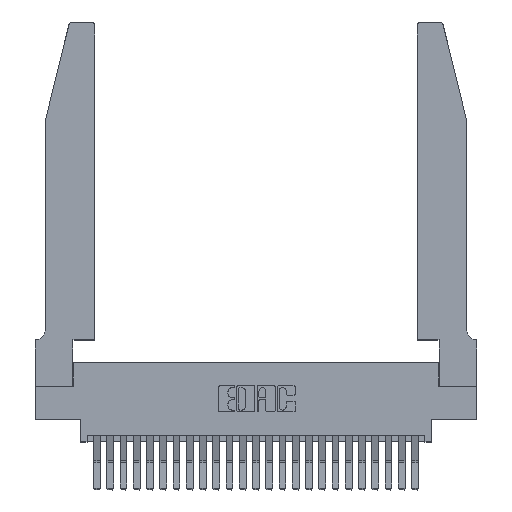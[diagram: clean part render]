
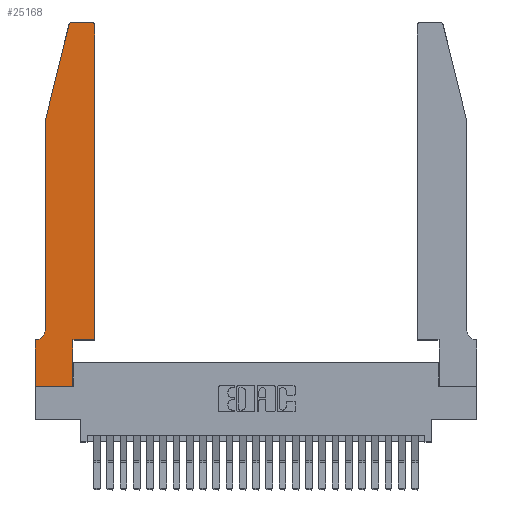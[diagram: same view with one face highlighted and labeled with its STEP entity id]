
A CAD part, top view. The second image highlights one B-rep face of the part: STEP entity #25168.
In plain terms, the highlighted planar face has unit normal (0, 0, 1).
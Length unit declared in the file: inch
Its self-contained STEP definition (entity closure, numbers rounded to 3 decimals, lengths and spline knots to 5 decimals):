
#129 = ORIENTED_EDGE ( 'NONE', *, *, #20044, .T. ) ;
#141 = EDGE_CURVE ( 'NONE', #10245, #15289, #26873, .T. ) ;
#206 = VERTEX_POINT ( 'NONE', #9974 ) ;
#524 = VERTEX_POINT ( 'NONE', #25598 ) ;
#725 = DIRECTION ( 'NONE',  ( 0., -1., 0. ) ) ;
#906 = LINE ( 'NONE', #17146, #22350 ) ;
#1101 = DIRECTION ( 'NONE',  ( 1., 0., 0. ) ) ;
#1285 = CARTESIAN_POINT ( 'NONE',  ( 0., 0., 0.37 ) ) ;
#1802 = DIRECTION ( 'NONE',  ( 1., 0., 0. ) ) ;
#1846 = DIRECTION ( 'NONE',  ( 1., 0., 0. ) ) ;
#2119 = DIRECTION ( 'NONE',  ( 1., 0., 0. ) ) ;
#2257 = VERTEX_POINT ( 'NONE', #11259 ) ;
#2461 = VERTEX_POINT ( 'NONE', #10175 ) ;
#2646 = CARTESIAN_POINT ( 'NONE',  ( 0.2865, 0.35, 0.37 ) ) ;
#2958 = DIRECTION ( 'NONE',  ( 0., -1., 0. ) ) ;
#3102 = LINE ( 'NONE', #10733, #10569 ) ;
#3247 = DIRECTION ( 'NONE',  ( 0., 0., -1. ) ) ;
#3301 = VECTOR ( 'NONE', #19074, 39.37008 ) ;
#3328 = DIRECTION ( 'NONE',  ( -1., 0., 0. ) ) ;
#3573 = ORIENTED_EDGE ( 'NONE', *, *, #22292, .T. ) ;
#4058 = CARTESIAN_POINT ( 'NONE',  ( 0.2865, 0., 0.37 ) ) ;
#4176 = CARTESIAN_POINT ( 'NONE',  ( 0.284, 2.72, 0.37 ) ) ;
#4724 = DIRECTION ( 'NONE',  ( -1., 0., 0. ) ) ;
#5297 = EDGE_CURVE ( 'NONE', #2461, #15305, #26559, .T. ) ;
#6252 = DIRECTION ( 'NONE',  ( 0., 0., 1. ) ) ;
#6571 = LINE ( 'NONE', #19351, #14093 ) ;
#6821 = CARTESIAN_POINT ( 'NONE',  ( 0.0755, 2., 0.37 ) ) ;
#8067 = AXIS2_PLACEMENT_3D ( 'NONE', #9018, #15135, #12956 ) ;
#8421 = ORIENTED_EDGE ( 'NONE', *, *, #18943, .T. ) ;
#8515 = CIRCLE ( 'NONE', #12895, 0.03 ) ;
#8526 = ORIENTED_EDGE ( 'NONE', *, *, #15415, .T. ) ;
#9018 = CARTESIAN_POINT ( 'NONE',  ( 0., 0.35, 0.37 ) ) ;
#9131 = CARTESIAN_POINT ( 'NONE',  ( 0.4505, 0.35, 0.37 ) ) ;
#9262 = DIRECTION ( 'NONE',  ( -0.239, -0.971, 0. ) ) ;
#9376 = CARTESIAN_POINT ( 'NONE',  ( 0.0755, 2., 0.37 ) ) ;
#9525 = CARTESIAN_POINT ( 'NONE',  ( 0.4205, 2.72, 0.37 ) ) ;
#9974 = CARTESIAN_POINT ( 'NONE',  ( 0.4505, 2.72, 0.37 ) ) ;
#10175 = CARTESIAN_POINT ( 'NONE',  ( 0.25487, 2.72718, 0.37 ) ) ;
#10245 = VERTEX_POINT ( 'NONE', #1285 ) ;
#10316 = VERTEX_POINT ( 'NONE', #25135 ) ;
#10436 = ORIENTED_EDGE ( 'NONE', *, *, #25226, .T. ) ;
#10569 = VECTOR ( 'NONE', #17134, 39.37008 ) ;
#10733 = CARTESIAN_POINT ( 'NONE',  ( 0.2605, 2.75, 0.37 ) ) ;
#10948 = CARTESIAN_POINT ( 'NONE',  ( 0.0055, 0.35, 0.37 ) ) ;
#11096 = CARTESIAN_POINT ( 'NONE',  ( 0.4205, 2.75, 0.37 ) ) ;
#11259 = CARTESIAN_POINT ( 'NONE',  ( 0.2865, 0.35, 0.37 ) ) ;
#11508 = CARTESIAN_POINT ( 'NONE',  ( 0.0055, 0.42, 0.37 ) ) ;
#11611 = VECTOR ( 'NONE', #1802, 39.37008 ) ;
#12684 = CARTESIAN_POINT ( 'NONE',  ( 0.284, 2.75, 0.37 ) ) ;
#12704 = EDGE_CURVE ( 'NONE', #206, #19803, #8515, .T. ) ;
#12749 = FACE_OUTER_BOUND ( 'NONE', #19467, .T. ) ;
#12799 = LINE ( 'NONE', #18111, #26760 ) ;
#12869 = ORIENTED_EDGE ( 'NONE', *, *, #14591, .T. ) ;
#12895 = AXIS2_PLACEMENT_3D ( 'NONE', #9525, #13556, #1101 ) ;
#12956 = DIRECTION ( 'NONE',  ( 1., 0., 0. ) ) ;
#13161 = CARTESIAN_POINT ( 'NONE',  ( 0., 0., 0.37 ) ) ;
#13297 = EDGE_CURVE ( 'NONE', #15289, #2257, #25417, .T. ) ;
#13520 = EDGE_CURVE ( 'NONE', #24922, #2461, #23122, .T. ) ;
#13556 = DIRECTION ( 'NONE',  ( 0., 0., 1. ) ) ;
#13970 = LINE ( 'NONE', #13161, #23040 ) ;
#14066 = VECTOR ( 'NONE', #2958, 39.37008 ) ;
#14093 = VECTOR ( 'NONE', #21197, 39.37008 ) ;
#14591 = EDGE_CURVE ( 'NONE', #524, #17059, #24705, .T. ) ;
#14635 = CARTESIAN_POINT ( 'NONE',  ( 0.0755, 2., 0.37 ) ) ;
#15135 = DIRECTION ( 'NONE',  ( 0., 0., 1. ) ) ;
#15289 = VERTEX_POINT ( 'NONE', #4058 ) ;
#15305 = VERTEX_POINT ( 'NONE', #14635 ) ;
#15415 = EDGE_CURVE ( 'NONE', #10316, #10245, #13970, .T. ) ;
#16596 = ORIENTED_EDGE ( 'NONE', *, *, #12704, .T. ) ;
#17059 = VERTEX_POINT ( 'NONE', #10948 ) ;
#17134 = DIRECTION ( 'NONE',  ( -1., 0., 0. ) ) ;
#17146 = CARTESIAN_POINT ( 'NONE',  ( 0.0755, 0.35, 0.37 ) ) ;
#18111 = CARTESIAN_POINT ( 'NONE',  ( 0.4505, 0.35, 0.37 ) ) ;
#18943 = EDGE_CURVE ( 'NONE', #17059, #10316, #906, .T. ) ;
#19074 = DIRECTION ( 'NONE',  ( 0., 1., 0. ) ) ;
#19133 = PLANE ( 'NONE',  #8067 ) ;
#19351 = CARTESIAN_POINT ( 'NONE',  ( 0.4505, 0.35, 0.37 ) ) ;
#19467 = EDGE_LOOP ( 'NONE', ( #129, #24214, #21488, #10436, #12869, #8421, #8526, #25170, #24361, #20760, #3573, #16596 ) ) ;
#19803 = VERTEX_POINT ( 'NONE', #11096 ) ;
#20044 = EDGE_CURVE ( 'NONE', #19803, #24922, #3102, .T. ) ;
#20334 = CARTESIAN_POINT ( 'NONE',  ( 0., 0., 0.37 ) ) ;
#20760 = ORIENTED_EDGE ( 'NONE', *, *, #21231, .T. ) ;
#21197 = DIRECTION ( 'NONE',  ( 0., 1., 0. ) ) ;
#21231 = EDGE_CURVE ( 'NONE', #2257, #21881, #12799, .T. ) ;
#21488 = ORIENTED_EDGE ( 'NONE', *, *, #5297, .T. ) ;
#21881 = VERTEX_POINT ( 'NONE', #9131 ) ;
#22292 = EDGE_CURVE ( 'NONE', #21881, #206, #6571, .T. ) ;
#22350 = VECTOR ( 'NONE', #4724, 39.37008 ) ;
#22477 = AXIS2_PLACEMENT_3D ( 'NONE', #4176, #6252, #2119 ) ;
#23040 = VECTOR ( 'NONE', #725, 39.37008 ) ;
#23122 = CIRCLE ( 'NONE', #22477, 0.03 ) ;
#23154 = LINE ( 'NONE', #9376, #14066 ) ;
#23948 = VECTOR ( 'NONE', #9262, 39.37008 ) ;
#24031 = AXIS2_PLACEMENT_3D ( 'NONE', #11508, #3247, #3328 ) ;
#24214 = ORIENTED_EDGE ( 'NONE', *, *, #13520, .T. ) ;
#24361 = ORIENTED_EDGE ( 'NONE', *, *, #13297, .T. ) ;
#24705 = CIRCLE ( 'NONE', #24031, 0.07 ) ;
#24922 = VERTEX_POINT ( 'NONE', #12684 ) ;
#25135 = CARTESIAN_POINT ( 'NONE',  ( 0., 0.35, 0.37 ) ) ;
#25168 = ADVANCED_FACE ( 'NONE', ( #12749 ), #19133, .T. ) ;
#25170 = ORIENTED_EDGE ( 'NONE', *, *, #141, .T. ) ;
#25226 = EDGE_CURVE ( 'NONE', #15305, #524, #23154, .T. ) ;
#25417 = LINE ( 'NONE', #2646, #3301 ) ;
#25598 = CARTESIAN_POINT ( 'NONE',  ( 0.0755, 0.42, 0.37 ) ) ;
#26559 = LINE ( 'NONE', #6821, #23948 ) ;
#26760 = VECTOR ( 'NONE', #1846, 39.37008 ) ;
#26873 = LINE ( 'NONE', #20334, #11611 ) ;
